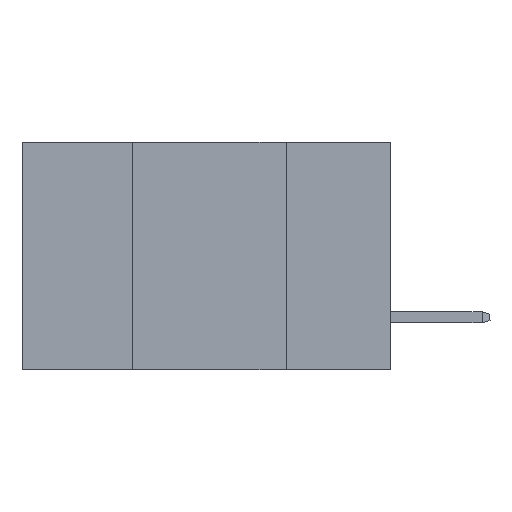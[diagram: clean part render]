
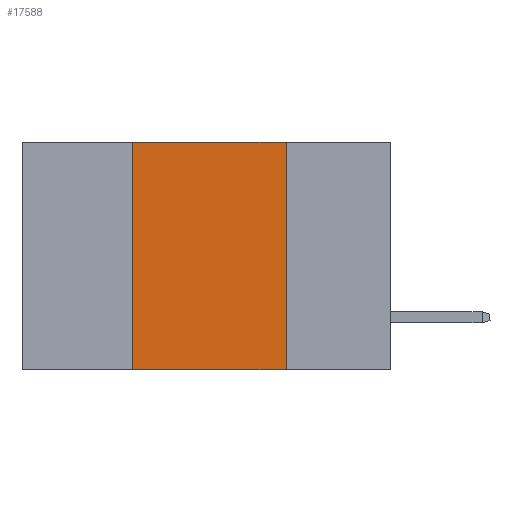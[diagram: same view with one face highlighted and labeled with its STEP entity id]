
A CAD part, left-side view. The second image highlights one B-rep face of the part: STEP entity #17588.
In plain terms, the highlighted planar face has unit normal (-1, 0, 0).
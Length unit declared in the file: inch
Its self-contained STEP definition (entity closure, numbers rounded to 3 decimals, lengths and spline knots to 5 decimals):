
#380 = EDGE_CURVE ( 'NONE', #19343, #14009, #18053, .T. ) ;
#2379 = CARTESIAN_POINT ( 'NONE',  ( 0., 0.42, 0. ) ) ;
#2724 = EDGE_LOOP ( 'NONE', ( #20490, #7229, #4158, #11471 ) ) ;
#4158 = ORIENTED_EDGE ( 'NONE', *, *, #8349, .F. ) ;
#4853 = CARTESIAN_POINT ( 'NONE',  ( 0., 0.6, -0.37 ) ) ;
#5727 = CARTESIAN_POINT ( 'NONE',  ( 0., 0.17, -0.37 ) ) ;
#6107 = VECTOR ( 'NONE', #10248, 39.37008 ) ;
#6665 = LINE ( 'NONE', #14740, #24710 ) ;
#7229 = ORIENTED_EDGE ( 'NONE', *, *, #22693, .F. ) ;
#7685 = DIRECTION ( 'NONE',  ( 0., -1., 0. ) ) ;
#8323 = CARTESIAN_POINT ( 'NONE',  ( 0., 0.42, 0. ) ) ;
#8349 = EDGE_CURVE ( 'NONE', #15613, #22575, #28202, .T. ) ;
#8784 = AXIS2_PLACEMENT_3D ( 'NONE', #12623, #28953, #15052 ) ;
#10248 = DIRECTION ( 'NONE',  ( 0., 0., -1. ) ) ;
#11471 = ORIENTED_EDGE ( 'NONE', *, *, #29701, .T. ) ;
#11657 = LINE ( 'NONE', #4853, #23440 ) ;
#12623 = CARTESIAN_POINT ( 'NONE',  ( 0., 0.6, 0. ) ) ;
#14009 = VERTEX_POINT ( 'NONE', #5727 ) ;
#14740 = CARTESIAN_POINT ( 'NONE',  ( 0., 0.6, 0. ) ) ;
#15052 = DIRECTION ( 'NONE',  ( 0., 0., -1. ) ) ;
#15613 = VERTEX_POINT ( 'NONE', #25856 ) ;
#17588 = ADVANCED_FACE ( 'NONE', ( #23937 ), #22034, .F. ) ;
#18053 = LINE ( 'NONE', #23801, #6107 ) ;
#19343 = VERTEX_POINT ( 'NONE', #21064 ) ;
#20490 = ORIENTED_EDGE ( 'NONE', *, *, #380, .F. ) ;
#21064 = CARTESIAN_POINT ( 'NONE',  ( 0., 0.17, 0. ) ) ;
#22034 = PLANE ( 'NONE',  #8784 ) ;
#22452 = DIRECTION ( 'NONE',  ( 0., 0., 1. ) ) ;
#22575 = VERTEX_POINT ( 'NONE', #2379 ) ;
#22693 = EDGE_CURVE ( 'NONE', #22575, #19343, #6665, .T. ) ;
#23440 = VECTOR ( 'NONE', #23772, 39.37008 ) ;
#23772 = DIRECTION ( 'NONE',  ( 0., -1., 0. ) ) ;
#23801 = CARTESIAN_POINT ( 'NONE',  ( 0., 0.17, 0. ) ) ;
#23937 = FACE_OUTER_BOUND ( 'NONE', #2724, .T. ) ;
#24710 = VECTOR ( 'NONE', #7685, 39.37008 ) ;
#25856 = CARTESIAN_POINT ( 'NONE',  ( 0., 0.42, -0.37 ) ) ;
#27482 = VECTOR ( 'NONE', #22452, 39.37008 ) ;
#28202 = LINE ( 'NONE', #8323, #27482 ) ;
#28953 = DIRECTION ( 'NONE',  ( 1., 0., 0. ) ) ;
#29701 = EDGE_CURVE ( 'NONE', #15613, #14009, #11657, .T. ) ;
